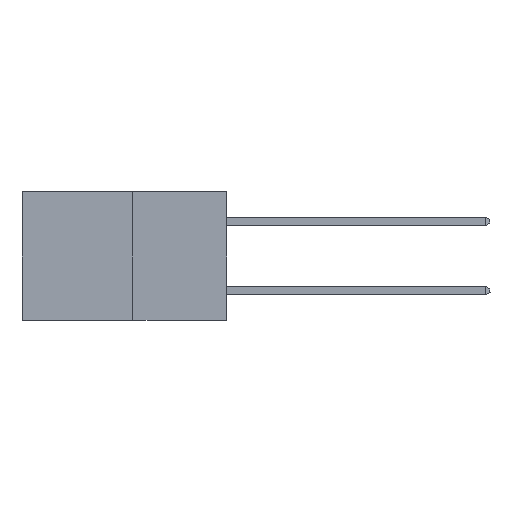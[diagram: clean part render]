
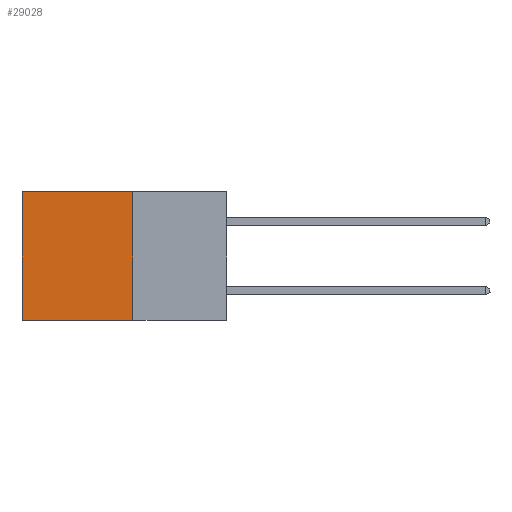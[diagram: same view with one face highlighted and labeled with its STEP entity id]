
A CAD part, left-side view. The second image highlights one B-rep face of the part: STEP entity #29028.
In plain terms, the highlighted planar face has unit normal (-1, 0, 0).
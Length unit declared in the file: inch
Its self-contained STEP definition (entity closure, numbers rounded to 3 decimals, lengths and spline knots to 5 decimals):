
#1102 = VECTOR ( 'NONE', #18787, 39.37008 ) ;
#1138 = ORIENTED_EDGE ( 'NONE', *, *, #17519, .F. ) ;
#1266 = DIRECTION ( 'NONE',  ( 0., 0., -1. ) ) ;
#2090 = DIRECTION ( 'NONE',  ( 1., 0., 0. ) ) ;
#4260 = VECTOR ( 'NONE', #1266, 39.37008 ) ;
#4526 = EDGE_CURVE ( 'NONE', #7999, #26998, #12742, .T. ) ;
#4558 = VERTEX_POINT ( 'NONE', #25063 ) ;
#6294 = EDGE_LOOP ( 'NONE', ( #23343, #18755, #1138, #14158 ) ) ;
#6562 = VECTOR ( 'NONE', #24050, 39.37008 ) ;
#6910 = VERTEX_POINT ( 'NONE', #18869 ) ;
#7999 = VERTEX_POINT ( 'NONE', #20322 ) ;
#11562 = LINE ( 'NONE', #17214, #22854 ) ;
#12093 = CARTESIAN_POINT ( 'NONE',  ( 0.277, 0.27, 0. ) ) ;
#12742 = LINE ( 'NONE', #12093, #1102 ) ;
#12799 = DIRECTION ( 'NONE',  ( 0., 1., 0. ) ) ;
#14158 = ORIENTED_EDGE ( 'NONE', *, *, #4526, .T. ) ;
#15070 = CARTESIAN_POINT ( 'NONE',  ( 0.277, 0.27, -0.37 ) ) ;
#15893 = CARTESIAN_POINT ( 'NONE',  ( 0.277, 0.27, -0.37 ) ) ;
#16098 = CARTESIAN_POINT ( 'NONE',  ( 0.277, 0.59, 0. ) ) ;
#17214 = CARTESIAN_POINT ( 'NONE',  ( 0.277, 0.27, -0.37 ) ) ;
#17519 = EDGE_CURVE ( 'NONE', #7999, #6910, #19384, .T. ) ;
#18174 = DIRECTION ( 'NONE',  ( 0., 0., -1. ) ) ;
#18207 = EDGE_CURVE ( 'NONE', #6910, #4558, #11562, .T. ) ;
#18755 = ORIENTED_EDGE ( 'NONE', *, *, #18207, .F. ) ;
#18787 = DIRECTION ( 'NONE',  ( 0., 1., 0. ) ) ;
#18869 = CARTESIAN_POINT ( 'NONE',  ( 0.277, 0.27, -0.37 ) ) ;
#18890 = EDGE_CURVE ( 'NONE', #26998, #4558, #22453, .T. ) ;
#19384 = LINE ( 'NONE', #15070, #6562 ) ;
#19456 = CARTESIAN_POINT ( 'NONE',  ( 0.277, 0.59, -0.37 ) ) ;
#20322 = CARTESIAN_POINT ( 'NONE',  ( 0.277, 0.27, 0. ) ) ;
#21101 = AXIS2_PLACEMENT_3D ( 'NONE', #15893, #2090, #18174 ) ;
#22453 = LINE ( 'NONE', #19456, #4260 ) ;
#22854 = VECTOR ( 'NONE', #12799, 39.37008 ) ;
#23343 = ORIENTED_EDGE ( 'NONE', *, *, #18890, .T. ) ;
#24050 = DIRECTION ( 'NONE',  ( 0., 0., -1. ) ) ;
#24137 = FACE_OUTER_BOUND ( 'NONE', #6294, .T. ) ;
#25063 = CARTESIAN_POINT ( 'NONE',  ( 0.277, 0.59, -0.37 ) ) ;
#26998 = VERTEX_POINT ( 'NONE', #16098 ) ;
#29028 = ADVANCED_FACE ( 'NONE', ( #24137 ), #29355, .F. ) ;
#29355 = PLANE ( 'NONE',  #21101 ) ;
